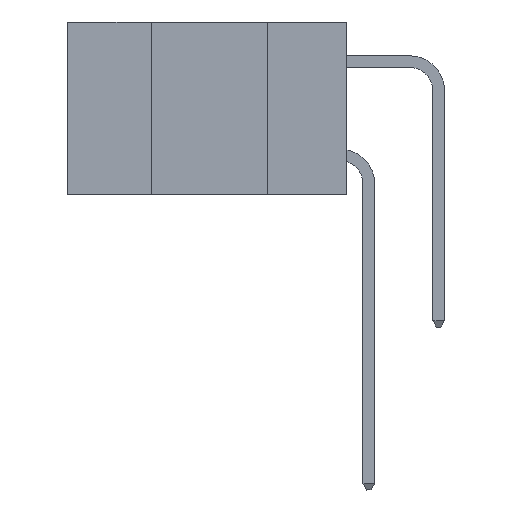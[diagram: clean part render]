
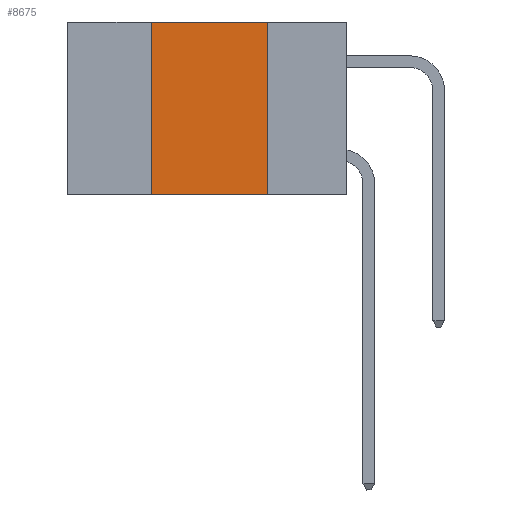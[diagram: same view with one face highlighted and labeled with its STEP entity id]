
A CAD part, left-side view. The second image highlights one B-rep face of the part: STEP entity #8675.
In plain terms, the highlighted planar face has unit normal (-1, 0, 0).
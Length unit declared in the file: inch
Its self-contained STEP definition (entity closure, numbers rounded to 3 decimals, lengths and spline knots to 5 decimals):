
#1637 = VECTOR ( 'NONE', #20243, 39.37008 ) ;
#1749 = DIRECTION ( 'NONE',  ( 0., 0., 1. ) ) ;
#2585 = CARTESIAN_POINT ( 'NONE',  ( 0., 0.17, 0. ) ) ;
#3131 = CARTESIAN_POINT ( 'NONE',  ( 0., 0.6, 0. ) ) ;
#3206 = EDGE_LOOP ( 'NONE', ( #31032, #30919, #17784, #28855 ) ) ;
#5227 = EDGE_CURVE ( 'NONE', #6555, #11441, #9531, .T. ) ;
#5902 = LINE ( 'NONE', #24295, #9624 ) ;
#6555 = VERTEX_POINT ( 'NONE', #22681 ) ;
#7099 = VERTEX_POINT ( 'NONE', #16130 ) ;
#7183 = VERTEX_POINT ( 'NONE', #7713 ) ;
#7713 = CARTESIAN_POINT ( 'NONE',  ( 0., 0.17, -0.37 ) ) ;
#8516 = CARTESIAN_POINT ( 'NONE',  ( 0., 0.6, 0. ) ) ;
#8675 = ADVANCED_FACE ( 'NONE', ( #13806 ), #26623, .F. ) ;
#9531 = LINE ( 'NONE', #8516, #19669 ) ;
#9624 = VECTOR ( 'NONE', #24025, 39.37008 ) ;
#11441 = VERTEX_POINT ( 'NONE', #13689 ) ;
#11650 = DIRECTION ( 'NONE',  ( 0., -1., 0. ) ) ;
#12179 = AXIS2_PLACEMENT_3D ( 'NONE', #3131, #23433, #15120 ) ;
#13689 = CARTESIAN_POINT ( 'NONE',  ( 0., 0.17, 0. ) ) ;
#13806 = FACE_OUTER_BOUND ( 'NONE', #3206, .T. ) ;
#15120 = DIRECTION ( 'NONE',  ( 0., 0., -1. ) ) ;
#15656 = EDGE_CURVE ( 'NONE', #7099, #6555, #30153, .T. ) ;
#16130 = CARTESIAN_POINT ( 'NONE',  ( 0., 0.42, -0.37 ) ) ;
#17784 = ORIENTED_EDGE ( 'NONE', *, *, #15656, .F. ) ;
#19669 = VECTOR ( 'NONE', #11650, 39.37008 ) ;
#20243 = DIRECTION ( 'NONE',  ( 0., 0., -1. ) ) ;
#22681 = CARTESIAN_POINT ( 'NONE',  ( 0., 0.42, 0. ) ) ;
#23333 = EDGE_CURVE ( 'NONE', #7099, #7183, #5902, .T. ) ;
#23433 = DIRECTION ( 'NONE',  ( 1., 0., 0. ) ) ;
#24025 = DIRECTION ( 'NONE',  ( 0., -1., 0. ) ) ;
#24295 = CARTESIAN_POINT ( 'NONE',  ( 0., 0.6, -0.37 ) ) ;
#25070 = EDGE_CURVE ( 'NONE', #11441, #7183, #25562, .T. ) ;
#25562 = LINE ( 'NONE', #2585, #1637 ) ;
#26623 = PLANE ( 'NONE',  #12179 ) ;
#28855 = ORIENTED_EDGE ( 'NONE', *, *, #23333, .T. ) ;
#30153 = LINE ( 'NONE', #34085, #32026 ) ;
#30919 = ORIENTED_EDGE ( 'NONE', *, *, #5227, .F. ) ;
#31032 = ORIENTED_EDGE ( 'NONE', *, *, #25070, .F. ) ;
#32026 = VECTOR ( 'NONE', #1749, 39.37008 ) ;
#34085 = CARTESIAN_POINT ( 'NONE',  ( 0., 0.42, 0. ) ) ;
